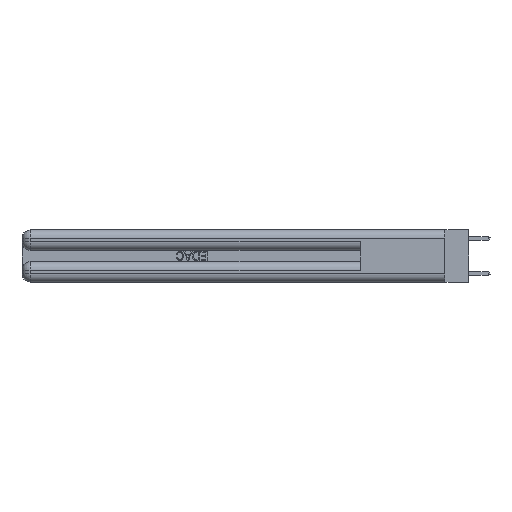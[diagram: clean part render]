
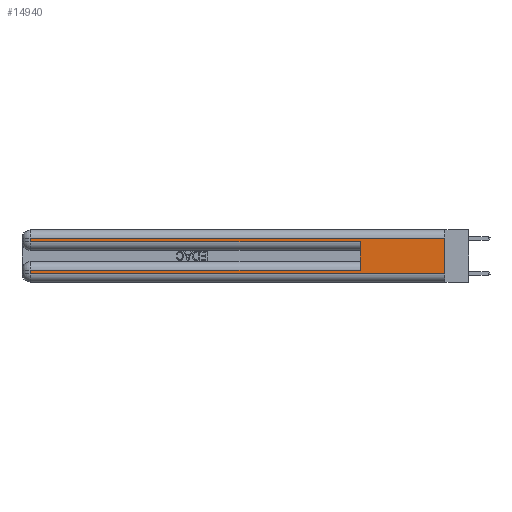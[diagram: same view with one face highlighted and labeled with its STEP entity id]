
A CAD part, left-side view. The second image highlights one B-rep face of the part: STEP entity #14940.
In plain terms, the highlighted planar face has unit normal (-1, 0, 0).
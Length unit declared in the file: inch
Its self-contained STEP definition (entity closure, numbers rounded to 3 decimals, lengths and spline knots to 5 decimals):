
#438 = CARTESIAN_POINT ( 'NONE',  ( 0., 0., 0.31 ) ) ;
#2742 = CARTESIAN_POINT ( 'NONE',  ( 0., 0., 0.31 ) ) ;
#3301 = CARTESIAN_POINT ( 'NONE',  ( 0., 2.94, 0.37 ) ) ;
#3690 = EDGE_CURVE ( 'NONE', #16732, #26807, #15469, .T. ) ;
#4213 = ORIENTED_EDGE ( 'NONE', *, *, #21358, .F. ) ;
#4684 = ORIENTED_EDGE ( 'NONE', *, *, #15108, .T. ) ;
#5032 = CARTESIAN_POINT ( 'NONE',  ( 0., 0.6, 0.285 ) ) ;
#5352 = EDGE_LOOP ( 'NONE', ( #25952, #4684, #5754, #19320, #4213, #18238, #7306, #23644 ) ) ;
#5754 = ORIENTED_EDGE ( 'NONE', *, *, #23199, .T. ) ;
#6041 = CARTESIAN_POINT ( 'NONE',  ( 0., 0., 0.06 ) ) ;
#6381 = EDGE_CURVE ( 'NONE', #22330, #16732, #20602, .T. ) ;
#7043 = VECTOR ( 'NONE', #25386, 39.37008 ) ;
#7306 = ORIENTED_EDGE ( 'NONE', *, *, #6381, .T. ) ;
#7503 = VERTEX_POINT ( 'NONE', #25378 ) ;
#7513 = LINE ( 'NONE', #18224, #13499 ) ;
#7872 = AXIS2_PLACEMENT_3D ( 'NONE', #20046, #22068, #12826 ) ;
#9030 = CARTESIAN_POINT ( 'NONE',  ( 0., 2.94, 0.085 ) ) ;
#9112 = VECTOR ( 'NONE', #27853, 39.37008 ) ;
#9354 = DIRECTION ( 'NONE',  ( 0., 1., 0. ) ) ;
#10109 = CARTESIAN_POINT ( 'NONE',  ( 0., 0., 0.085 ) ) ;
#10333 = EDGE_CURVE ( 'NONE', #26253, #17234, #7513, .T. ) ;
#10570 = EDGE_CURVE ( 'NONE', #13167, #22330, #12267, .T. ) ;
#10845 = LINE ( 'NONE', #21379, #25598 ) ;
#11542 = VECTOR ( 'NONE', #11792, 39.37008 ) ;
#11792 = DIRECTION ( 'NONE',  ( 0., 0., -1. ) ) ;
#12267 = LINE ( 'NONE', #10109, #24121 ) ;
#12826 = DIRECTION ( 'NONE',  ( 0., 0., -1. ) ) ;
#13167 = VERTEX_POINT ( 'NONE', #23836 ) ;
#13499 = VECTOR ( 'NONE', #27045, 39.37008 ) ;
#13981 = CARTESIAN_POINT ( 'NONE',  ( 0., 2.94, 0.37 ) ) ;
#14940 = ADVANCED_FACE ( 'NONE', ( #19766 ), #24390, .F. ) ;
#15108 = EDGE_CURVE ( 'NONE', #16992, #7503, #15738, .T. ) ;
#15469 = LINE ( 'NONE', #28503, #24793 ) ;
#15738 = LINE ( 'NONE', #2742, #26811 ) ;
#16732 = VERTEX_POINT ( 'NONE', #24067 ) ;
#16992 = VERTEX_POINT ( 'NONE', #438 ) ;
#17234 = VERTEX_POINT ( 'NONE', #5032 ) ;
#17328 = CARTESIAN_POINT ( 'NONE',  ( 0., 2.94, 0.285 ) ) ;
#18224 = CARTESIAN_POINT ( 'NONE',  ( 0., 0., 0.285 ) ) ;
#18238 = ORIENTED_EDGE ( 'NONE', *, *, #10570, .T. ) ;
#18863 = LINE ( 'NONE', #13981, #7043 ) ;
#18914 = DIRECTION ( 'NONE',  ( 0., 1., 0. ) ) ;
#19320 = ORIENTED_EDGE ( 'NONE', *, *, #10333, .T. ) ;
#19766 = FACE_OUTER_BOUND ( 'NONE', #5352, .T. ) ;
#20046 = CARTESIAN_POINT ( 'NONE',  ( 0., 0., 0.37 ) ) ;
#20602 = LINE ( 'NONE', #3301, #11542 ) ;
#21358 = EDGE_CURVE ( 'NONE', #13167, #17234, #10845, .T. ) ;
#21379 = CARTESIAN_POINT ( 'NONE',  ( 0., 0.6, 0.145 ) ) ;
#21614 = CARTESIAN_POINT ( 'NONE',  ( 0., 0., 0.37 ) ) ;
#21815 = DIRECTION ( 'NONE',  ( 0., 0., 1. ) ) ;
#22068 = DIRECTION ( 'NONE',  ( 1., 0., 0. ) ) ;
#22330 = VERTEX_POINT ( 'NONE', #9030 ) ;
#23199 = EDGE_CURVE ( 'NONE', #7503, #26253, #18863, .T. ) ;
#23644 = ORIENTED_EDGE ( 'NONE', *, *, #3690, .T. ) ;
#23836 = CARTESIAN_POINT ( 'NONE',  ( 0., 0.6, 0.085 ) ) ;
#24067 = CARTESIAN_POINT ( 'NONE',  ( 0., 2.94, 0.06 ) ) ;
#24073 = LINE ( 'NONE', #21614, #9112 ) ;
#24119 = DIRECTION ( 'NONE',  ( 0., -1., 0. ) ) ;
#24121 = VECTOR ( 'NONE', #18914, 39.37008 ) ;
#24390 = PLANE ( 'NONE',  #7872 ) ;
#24793 = VECTOR ( 'NONE', #24119, 39.37008 ) ;
#24839 = EDGE_CURVE ( 'NONE', #16992, #26807, #24073, .T. ) ;
#25378 = CARTESIAN_POINT ( 'NONE',  ( 0., 2.94, 0.31 ) ) ;
#25386 = DIRECTION ( 'NONE',  ( 0., 0., -1. ) ) ;
#25598 = VECTOR ( 'NONE', #21815, 39.37008 ) ;
#25952 = ORIENTED_EDGE ( 'NONE', *, *, #24839, .F. ) ;
#26253 = VERTEX_POINT ( 'NONE', #17328 ) ;
#26807 = VERTEX_POINT ( 'NONE', #6041 ) ;
#26811 = VECTOR ( 'NONE', #9354, 39.37008 ) ;
#27045 = DIRECTION ( 'NONE',  ( 0., -1., 0. ) ) ;
#27853 = DIRECTION ( 'NONE',  ( 0., 0., -1. ) ) ;
#28503 = CARTESIAN_POINT ( 'NONE',  ( 0., 0., 0.06 ) ) ;
